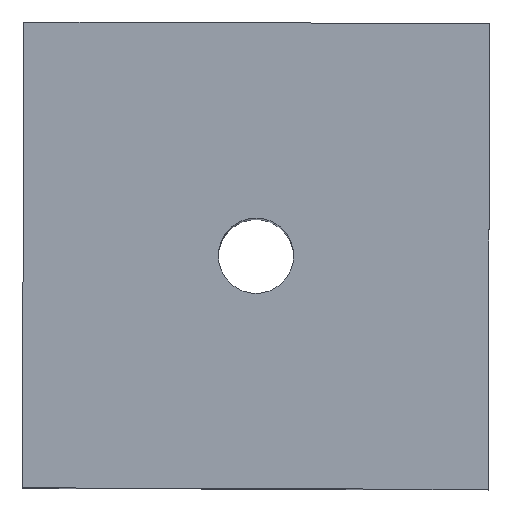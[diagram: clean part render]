
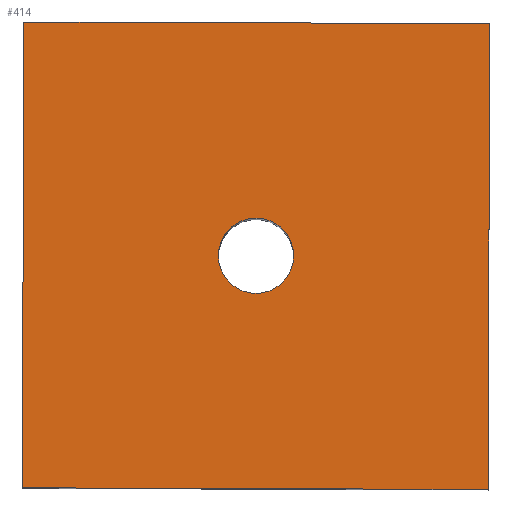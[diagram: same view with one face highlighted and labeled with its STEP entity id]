
A CAD part, top view. The second image highlights one B-rep face of the part: STEP entity #414.
In plain terms, the highlighted planar face has unit normal (0, 0, 1).
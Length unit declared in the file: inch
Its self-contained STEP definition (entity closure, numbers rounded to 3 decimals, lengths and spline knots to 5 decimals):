
#13 = CARTESIAN_POINT ( 'NONE',  ( -1.4375, 0.005, 5.5 ) ) ;
#34 = DIRECTION ( 'NONE',  ( 1., 0., 0. ) ) ;
#41 = AXIS2_PLACEMENT_3D ( 'NONE', #309, #375, #51 ) ;
#51 = DIRECTION ( 'NONE',  ( 1., 0., 0. ) ) ;
#63 = VECTOR ( 'NONE', #301, 39.37008 ) ;
#65 = DIRECTION ( 'NONE',  ( 0., 0., -1. ) ) ;
#75 = LINE ( 'NONE', #13, #63 ) ;
#76 = DIRECTION ( 'NONE',  ( 0.003, 1., 0. ) ) ;
#77 = EDGE_CURVE ( 'NONE', #96, #304, #221, .T. ) ;
#86 = DIRECTION ( 'NONE',  ( 1., -0.003, 0. ) ) ;
#88 = CARTESIAN_POINT ( 'NONE',  ( -1.4425, -1.4325, 5.5 ) ) ;
#96 = VERTEX_POINT ( 'NONE', #88 ) ;
#104 = CARTESIAN_POINT ( 'NONE',  ( 0.2325, 0., 5.5 ) ) ;
#121 = VERTEX_POINT ( 'NONE', #412 ) ;
#126 = CIRCLE ( 'NONE', #207, 0.2325 ) ;
#135 = DIRECTION ( 'NONE',  ( 1., 0., 0. ) ) ;
#139 = ORIENTED_EDGE ( 'NONE', *, *, #195, .T. ) ;
#159 = LINE ( 'NONE', #176, #180 ) ;
#161 = CIRCLE ( 'NONE', #185, 0.2325 ) ;
#165 = VERTEX_POINT ( 'NONE', #104 ) ;
#166 = EDGE_CURVE ( 'NONE', #165, #236, #161, .T. ) ;
#167 = VECTOR ( 'NONE', #179, 39.37008 ) ;
#176 = CARTESIAN_POINT ( 'NONE',  ( 1.4375, -0.005, 5.5 ) ) ;
#179 = DIRECTION ( 'NONE',  ( -1., 0.003, 0. ) ) ;
#180 = VECTOR ( 'NONE', #76, 39.37008 ) ;
#185 = AXIS2_PLACEMENT_3D ( 'NONE', #229, #325, #34 ) ;
#188 = FACE_OUTER_BOUND ( 'NONE', #254, .T. ) ;
#189 = PLANE ( 'NONE',  #41 ) ;
#195 = EDGE_CURVE ( 'NONE', #236, #165, #126, .T. ) ;
#207 = AXIS2_PLACEMENT_3D ( 'NONE', #293, #65, #135 ) ;
#209 = ORIENTED_EDGE ( 'NONE', *, *, #266, .T. ) ;
#216 = ORIENTED_EDGE ( 'NONE', *, *, #314, .T. ) ;
#221 = LINE ( 'NONE', #373, #368 ) ;
#223 = ORIENTED_EDGE ( 'NONE', *, *, #77, .T. ) ;
#229 = CARTESIAN_POINT ( 'NONE',  ( 0., 0., 5.5 ) ) ;
#236 = VERTEX_POINT ( 'NONE', #393 ) ;
#254 = EDGE_LOOP ( 'NONE', ( #223, #209, #383, #216 ) ) ;
#266 = EDGE_CURVE ( 'NONE', #304, #121, #159, .T. ) ;
#270 = CARTESIAN_POINT ( 'NONE',  ( 0.005, 1.4375, 5.5 ) ) ;
#275 = CARTESIAN_POINT ( 'NONE',  ( 1.4325, -1.4425, 5.5 ) ) ;
#283 = VERTEX_POINT ( 'NONE', #336 ) ;
#290 = ORIENTED_EDGE ( 'NONE', *, *, #166, .T. ) ;
#293 = CARTESIAN_POINT ( 'NONE',  ( 0., 0., 5.5 ) ) ;
#301 = DIRECTION ( 'NONE',  ( -0.003, -1., 0. ) ) ;
#304 = VERTEX_POINT ( 'NONE', #275 ) ;
#309 = CARTESIAN_POINT ( 'NONE',  ( 0., 0., 5.5 ) ) ;
#314 = EDGE_CURVE ( 'NONE', #283, #96, #75, .T. ) ;
#325 = DIRECTION ( 'NONE',  ( 0., 0., -1. ) ) ;
#328 = LINE ( 'NONE', #270, #167 ) ;
#336 = CARTESIAN_POINT ( 'NONE',  ( -1.4325, 1.4425, 5.5 ) ) ;
#368 = VECTOR ( 'NONE', #86, 39.37008 ) ;
#371 = FACE_BOUND ( 'NONE', #381, .T. ) ;
#373 = CARTESIAN_POINT ( 'NONE',  ( -0.005, -1.4375, 5.5 ) ) ;
#375 = DIRECTION ( 'NONE',  ( 0., 0., 1. ) ) ;
#378 = EDGE_CURVE ( 'NONE', #121, #283, #328, .T. ) ;
#381 = EDGE_LOOP ( 'NONE', ( #139, #290 ) ) ;
#383 = ORIENTED_EDGE ( 'NONE', *, *, #378, .T. ) ;
#393 = CARTESIAN_POINT ( 'NONE',  ( -0.2325, 0., 5.5 ) ) ;
#412 = CARTESIAN_POINT ( 'NONE',  ( 1.4425, 1.4325, 5.5 ) ) ;
#414 = ADVANCED_FACE ( 'NONE', ( #188, #371 ), #189, .T. ) ;
